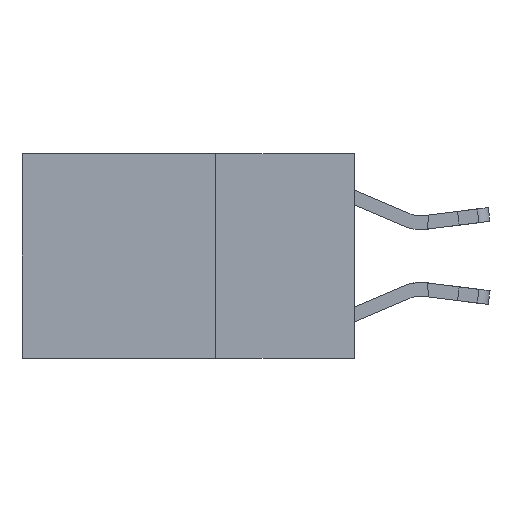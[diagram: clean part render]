
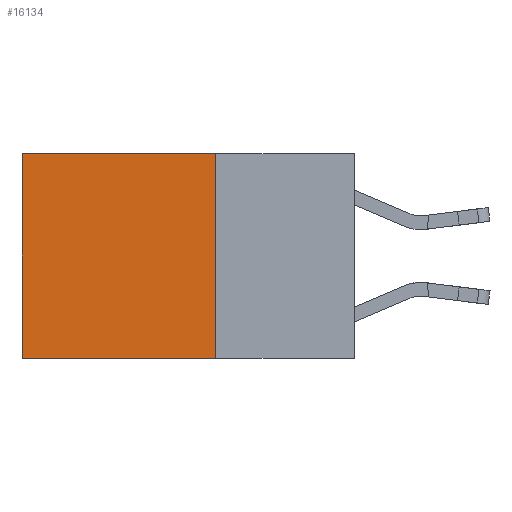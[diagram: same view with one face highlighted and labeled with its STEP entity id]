
A CAD part, left-side view. The second image highlights one B-rep face of the part: STEP entity #16134.
In plain terms, the highlighted planar face has unit normal (-1, 0, 0).
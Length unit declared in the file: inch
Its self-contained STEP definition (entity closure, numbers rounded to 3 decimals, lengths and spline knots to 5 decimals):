
#126 = CARTESIAN_POINT ( 'NONE',  ( 0.2625, 0.6, 0. ) ) ;
#390 = LINE ( 'NONE', #16786, #1426 ) ;
#1426 = VECTOR ( 'NONE', #6460, 39.37008 ) ;
#2066 = CARTESIAN_POINT ( 'NONE',  ( 0.2625, 0.25, -0.37 ) ) ;
#2202 = DIRECTION ( 'NONE',  ( 0., 0., -1. ) ) ;
#2622 = DIRECTION ( 'NONE',  ( 0., 0., -1. ) ) ;
#2952 = VERTEX_POINT ( 'NONE', #2066 ) ;
#4247 = VERTEX_POINT ( 'NONE', #11052 ) ;
#4948 = VERTEX_POINT ( 'NONE', #10189 ) ;
#6084 = PLANE ( 'NONE',  #15142 ) ;
#6460 = DIRECTION ( 'NONE',  ( 0., 1., 0. ) ) ;
#6711 = CARTESIAN_POINT ( 'NONE',  ( 0.2625, 0.6, 0. ) ) ;
#7053 = DIRECTION ( 'NONE',  ( 0., 1., 0. ) ) ;
#7554 = EDGE_CURVE ( 'NONE', #4247, #2952, #16797, .T. ) ;
#8873 = EDGE_CURVE ( 'NONE', #2952, #4948, #9650, .T. ) ;
#9396 = EDGE_CURVE ( 'NONE', #16357, #4948, #15761, .T. ) ;
#9453 = EDGE_LOOP ( 'NONE', ( #9667, #16004, #12844, #13935 ) ) ;
#9650 = LINE ( 'NONE', #11986, #15362 ) ;
#9667 = ORIENTED_EDGE ( 'NONE', *, *, #9396, .T. ) ;
#10189 = CARTESIAN_POINT ( 'NONE',  ( 0.2625, 0.6, -0.37 ) ) ;
#10745 = EDGE_CURVE ( 'NONE', #4247, #16357, #390, .T. ) ;
#10788 = FACE_OUTER_BOUND ( 'NONE', #9453, .T. ) ;
#11052 = CARTESIAN_POINT ( 'NONE',  ( 0.2625, 0.25, 0. ) ) ;
#11365 = CARTESIAN_POINT ( 'NONE',  ( 0.2625, 0.25, 0. ) ) ;
#11850 = CARTESIAN_POINT ( 'NONE',  ( 0.2625, 0.25, 0. ) ) ;
#11986 = CARTESIAN_POINT ( 'NONE',  ( 0.2625, 0.25, -0.37 ) ) ;
#12844 = ORIENTED_EDGE ( 'NONE', *, *, #7554, .F. ) ;
#13335 = VECTOR ( 'NONE', #14503, 39.37008 ) ;
#13935 = ORIENTED_EDGE ( 'NONE', *, *, #10745, .T. ) ;
#14503 = DIRECTION ( 'NONE',  ( 0., 0., -1. ) ) ;
#15142 = AXIS2_PLACEMENT_3D ( 'NONE', #11365, #16517, #2202 ) ;
#15362 = VECTOR ( 'NONE', #7053, 39.37008 ) ;
#15761 = LINE ( 'NONE', #126, #15964 ) ;
#15964 = VECTOR ( 'NONE', #2622, 39.37008 ) ;
#16004 = ORIENTED_EDGE ( 'NONE', *, *, #8873, .F. ) ;
#16134 = ADVANCED_FACE ( 'NONE', ( #10788 ), #6084, .F. ) ;
#16357 = VERTEX_POINT ( 'NONE', #6711 ) ;
#16517 = DIRECTION ( 'NONE',  ( 1., 0., 0. ) ) ;
#16786 = CARTESIAN_POINT ( 'NONE',  ( 0.2625, 0.25, 0. ) ) ;
#16797 = LINE ( 'NONE', #11850, #13335 ) ;
